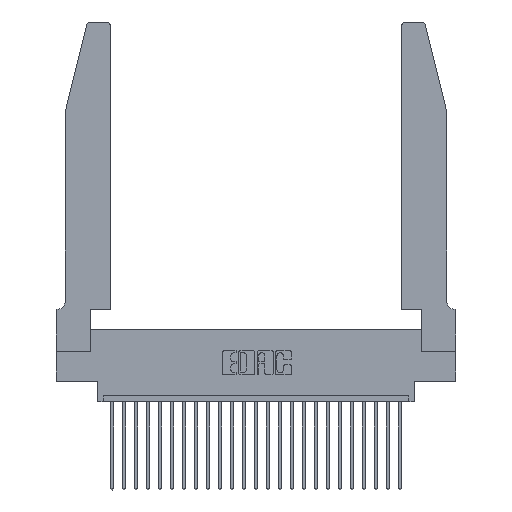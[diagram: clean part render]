
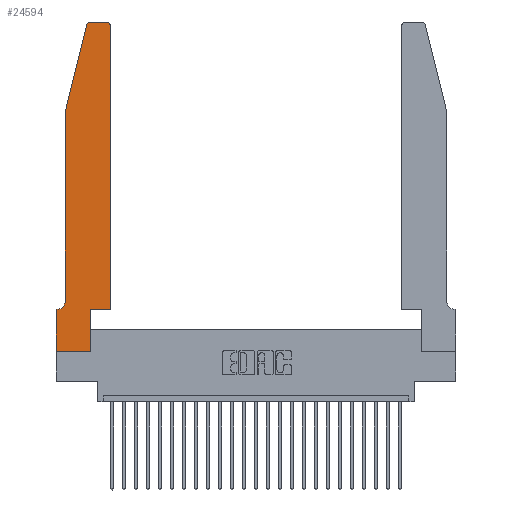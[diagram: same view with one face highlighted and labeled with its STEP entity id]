
A CAD part, top view. The second image highlights one B-rep face of the part: STEP entity #24594.
In plain terms, the highlighted planar face has unit normal (0, 0, 1).
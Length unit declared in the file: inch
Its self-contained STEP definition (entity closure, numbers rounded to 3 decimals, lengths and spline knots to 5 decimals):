
#41 = CARTESIAN_POINT ( 'NONE',  ( 0.284, 2.72, 0.37 ) ) ;
#230 = FACE_OUTER_BOUND ( 'NONE', #4479, .T. ) ;
#320 = VECTOR ( 'NONE', #22624, 39.37008 ) ;
#516 = ORIENTED_EDGE ( 'NONE', *, *, #16477, .T. ) ;
#639 = CIRCLE ( 'NONE', #4536, 0.07 ) ;
#1139 = EDGE_CURVE ( 'NONE', #18608, #4583, #14218, .T. ) ;
#1331 = CIRCLE ( 'NONE', #12332, 0.03 ) ;
#1360 = CARTESIAN_POINT ( 'NONE',  ( 0.2865, 0., 0.37 ) ) ;
#1461 = DIRECTION ( 'NONE',  ( 0., -1., 0. ) ) ;
#1820 = VECTOR ( 'NONE', #8231, 39.37008 ) ;
#2482 = CARTESIAN_POINT ( 'NONE',  ( 0., 0., 0.37 ) ) ;
#4479 = EDGE_LOOP ( 'NONE', ( #516, #14631, #9391, #9663, #20763, #24125, #21419, #21157, #4511, #15252, #5875, #25161 ) ) ;
#4511 = ORIENTED_EDGE ( 'NONE', *, *, #22487, .T. ) ;
#4536 = AXIS2_PLACEMENT_3D ( 'NONE', #23884, #21591, #7680 ) ;
#4583 = VERTEX_POINT ( 'NONE', #1360 ) ;
#4643 = LINE ( 'NONE', #5716, #20000 ) ;
#5716 = CARTESIAN_POINT ( 'NONE',  ( 0.0755, 2., 0.37 ) ) ;
#5875 = ORIENTED_EDGE ( 'NONE', *, *, #19022, .T. ) ;
#6362 = VECTOR ( 'NONE', #6552, 39.37008 ) ;
#6552 = DIRECTION ( 'NONE',  ( -1., 0., 0. ) ) ;
#6613 = CIRCLE ( 'NONE', #6801, 0.03 ) ;
#6792 = EDGE_CURVE ( 'NONE', #12588, #19791, #4643, .T. ) ;
#6801 = AXIS2_PLACEMENT_3D ( 'NONE', #41, #24295, #12223 ) ;
#7306 = CARTESIAN_POINT ( 'NONE',  ( 0.4205, 2.75, 0.37 ) ) ;
#7419 = CARTESIAN_POINT ( 'NONE',  ( 0.0755, 2., 0.37 ) ) ;
#7434 = CARTESIAN_POINT ( 'NONE',  ( 0.4505, 0.35, 0.37 ) ) ;
#7680 = DIRECTION ( 'NONE',  ( -1., 0., 0. ) ) ;
#7888 = DIRECTION ( 'NONE',  ( -1., 0., 0. ) ) ;
#8231 = DIRECTION ( 'NONE',  ( 0., -1., 0. ) ) ;
#8480 = DIRECTION ( 'NONE',  ( 1., 0., 0. ) ) ;
#8588 = EDGE_CURVE ( 'NONE', #9737, #21690, #10243, .T. ) ;
#8862 = EDGE_CURVE ( 'NONE', #25878, #12588, #18946, .T. ) ;
#9110 = LINE ( 'NONE', #16036, #1820 ) ;
#9391 = ORIENTED_EDGE ( 'NONE', *, *, #8862, .T. ) ;
#9515 = CARTESIAN_POINT ( 'NONE',  ( 0.0055, 0.35, 0.37 ) ) ;
#9663 = ORIENTED_EDGE ( 'NONE', *, *, #6792, .T. ) ;
#9678 = PLANE ( 'NONE',  #10310 ) ;
#9737 = VERTEX_POINT ( 'NONE', #10993 ) ;
#9769 = DIRECTION ( 'NONE',  ( 0., 0., 1. ) ) ;
#9849 = DIRECTION ( 'NONE',  ( 1., 0., 0. ) ) ;
#10053 = EDGE_CURVE ( 'NONE', #19791, #25513, #639, .T. ) ;
#10243 = LINE ( 'NONE', #17393, #11814 ) ;
#10310 = AXIS2_PLACEMENT_3D ( 'NONE', #21858, #9769, #9849 ) ;
#10332 = VERTEX_POINT ( 'NONE', #7306 ) ;
#10760 = CARTESIAN_POINT ( 'NONE',  ( 0.2865, 0.35, 0.37 ) ) ;
#10776 = LINE ( 'NONE', #16716, #6362 ) ;
#10993 = CARTESIAN_POINT ( 'NONE',  ( 0.2865, 0.35, 0.37 ) ) ;
#11121 = DIRECTION ( 'NONE',  ( -0.239, -0.971, 0. ) ) ;
#11814 = VECTOR ( 'NONE', #25503, 39.37008 ) ;
#12223 = DIRECTION ( 'NONE',  ( 1., 0., 0. ) ) ;
#12332 = AXIS2_PLACEMENT_3D ( 'NONE', #12779, #22678, #8480 ) ;
#12588 = VERTEX_POINT ( 'NONE', #7419 ) ;
#12779 = CARTESIAN_POINT ( 'NONE',  ( 0.4205, 2.72, 0.37 ) ) ;
#13103 = CARTESIAN_POINT ( 'NONE',  ( 0.284, 2.75, 0.37 ) ) ;
#14218 = LINE ( 'NONE', #2482, #320 ) ;
#14262 = EDGE_CURVE ( 'NONE', #15140, #10332, #1331, .T. ) ;
#14586 = VECTOR ( 'NONE', #11121, 39.37008 ) ;
#14631 = ORIENTED_EDGE ( 'NONE', *, *, #24650, .T. ) ;
#14950 = VERTEX_POINT ( 'NONE', #13103 ) ;
#15080 = CARTESIAN_POINT ( 'NONE',  ( 0.0755, 2., 0.37 ) ) ;
#15140 = VERTEX_POINT ( 'NONE', #15811 ) ;
#15252 = ORIENTED_EDGE ( 'NONE', *, *, #8588, .T. ) ;
#15654 = VECTOR ( 'NONE', #23744, 39.37008 ) ;
#15803 = VECTOR ( 'NONE', #7888, 39.37008 ) ;
#15811 = CARTESIAN_POINT ( 'NONE',  ( 0.4505, 2.72, 0.37 ) ) ;
#16036 = CARTESIAN_POINT ( 'NONE',  ( 0., 0., 0.37 ) ) ;
#16110 = EDGE_CURVE ( 'NONE', #25513, #20501, #16410, .T. ) ;
#16287 = CARTESIAN_POINT ( 'NONE',  ( 0.0755, 0.35, 0.37 ) ) ;
#16410 = LINE ( 'NONE', #16287, #15803 ) ;
#16477 = EDGE_CURVE ( 'NONE', #10332, #14950, #10776, .T. ) ;
#16716 = CARTESIAN_POINT ( 'NONE',  ( 0.2605, 2.75, 0.37 ) ) ;
#17393 = CARTESIAN_POINT ( 'NONE',  ( 0.4505, 0.35, 0.37 ) ) ;
#18085 = EDGE_CURVE ( 'NONE', #20501, #18608, #9110, .T. ) ;
#18608 = VERTEX_POINT ( 'NONE', #23803 ) ;
#18946 = LINE ( 'NONE', #15080, #14586 ) ;
#19022 = EDGE_CURVE ( 'NONE', #21690, #15140, #24725, .T. ) ;
#19113 = CARTESIAN_POINT ( 'NONE',  ( 0.0755, 0.42, 0.37 ) ) ;
#19791 = VERTEX_POINT ( 'NONE', #19113 ) ;
#20000 = VECTOR ( 'NONE', #1461, 39.37008 ) ;
#20501 = VERTEX_POINT ( 'NONE', #23203 ) ;
#20638 = DIRECTION ( 'NONE',  ( 0., 1., 0. ) ) ;
#20763 = ORIENTED_EDGE ( 'NONE', *, *, #10053, .T. ) ;
#20793 = LINE ( 'NONE', #10760, #24534 ) ;
#21028 = CARTESIAN_POINT ( 'NONE',  ( 0.4505, 0.35, 0.37 ) ) ;
#21157 = ORIENTED_EDGE ( 'NONE', *, *, #1139, .T. ) ;
#21419 = ORIENTED_EDGE ( 'NONE', *, *, #18085, .T. ) ;
#21591 = DIRECTION ( 'NONE',  ( 0., 0., -1. ) ) ;
#21690 = VERTEX_POINT ( 'NONE', #7434 ) ;
#21858 = CARTESIAN_POINT ( 'NONE',  ( 0., 0.35, 0.37 ) ) ;
#22487 = EDGE_CURVE ( 'NONE', #4583, #9737, #20793, .T. ) ;
#22624 = DIRECTION ( 'NONE',  ( 1., 0., 0. ) ) ;
#22678 = DIRECTION ( 'NONE',  ( 0., 0., 1. ) ) ;
#23203 = CARTESIAN_POINT ( 'NONE',  ( 0., 0.35, 0.37 ) ) ;
#23744 = DIRECTION ( 'NONE',  ( 0., 1., 0. ) ) ;
#23803 = CARTESIAN_POINT ( 'NONE',  ( 0., 0., 0.37 ) ) ;
#23884 = CARTESIAN_POINT ( 'NONE',  ( 0.0055, 0.42, 0.37 ) ) ;
#24125 = ORIENTED_EDGE ( 'NONE', *, *, #16110, .T. ) ;
#24295 = DIRECTION ( 'NONE',  ( 0., 0., 1. ) ) ;
#24457 = CARTESIAN_POINT ( 'NONE',  ( 0.25487, 2.72718, 0.37 ) ) ;
#24534 = VECTOR ( 'NONE', #20638, 39.37008 ) ;
#24594 = ADVANCED_FACE ( 'NONE', ( #230 ), #9678, .T. ) ;
#24650 = EDGE_CURVE ( 'NONE', #14950, #25878, #6613, .T. ) ;
#24725 = LINE ( 'NONE', #21028, #15654 ) ;
#25161 = ORIENTED_EDGE ( 'NONE', *, *, #14262, .T. ) ;
#25503 = DIRECTION ( 'NONE',  ( 1., 0., 0. ) ) ;
#25513 = VERTEX_POINT ( 'NONE', #9515 ) ;
#25878 = VERTEX_POINT ( 'NONE', #24457 ) ;
